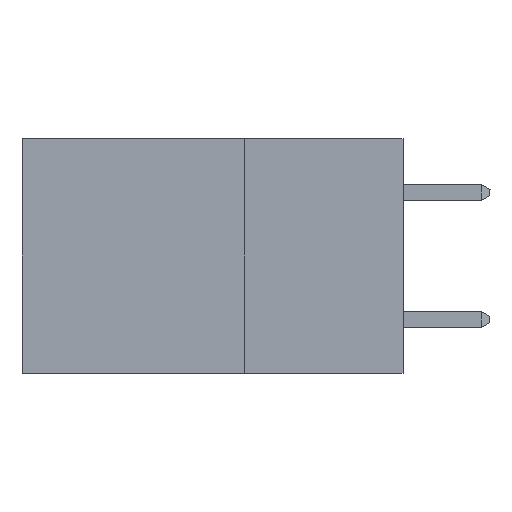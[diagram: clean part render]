
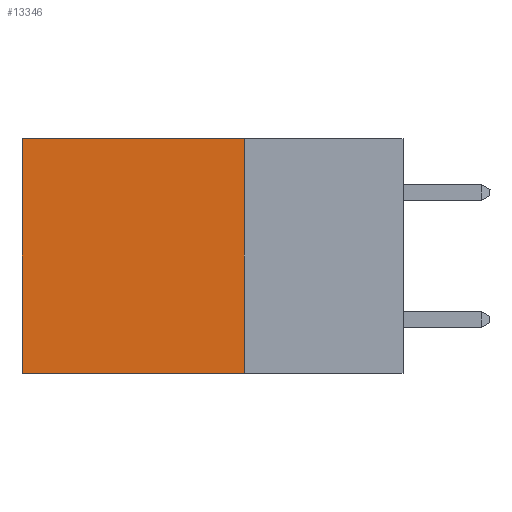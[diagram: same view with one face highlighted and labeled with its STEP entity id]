
A CAD part, left-side view. The second image highlights one B-rep face of the part: STEP entity #13346.
In plain terms, the highlighted planar face has unit normal (-1, 0, 0).
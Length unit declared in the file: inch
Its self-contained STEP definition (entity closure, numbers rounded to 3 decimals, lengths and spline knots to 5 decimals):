
#200 = LINE ( 'NONE', #30138, #27126 ) ;
#284 = LINE ( 'NONE', #18912, #17563 ) ;
#1075 = EDGE_CURVE ( 'NONE', #12666, #24099, #200, .T. ) ;
#2391 = CARTESIAN_POINT ( 'NONE',  ( 0.2875, 0.25, 0. ) ) ;
#2443 = CARTESIAN_POINT ( 'NONE',  ( 0.2875, 0.25, 0. ) ) ;
#2708 = CARTESIAN_POINT ( 'NONE',  ( 0.2875, 0.6, 0. ) ) ;
#4007 = FACE_OUTER_BOUND ( 'NONE', #5356, .T. ) ;
#4535 = VERTEX_POINT ( 'NONE', #2391 ) ;
#5356 = EDGE_LOOP ( 'NONE', ( #16468, #25986, #12578, #10674 ) ) ;
#5748 = VECTOR ( 'NONE', #8883, 39.37008 ) ;
#6306 = PLANE ( 'NONE',  #24813 ) ;
#8027 = CARTESIAN_POINT ( 'NONE',  ( 0.2875, 0.6, -0.37 ) ) ;
#8883 = DIRECTION ( 'NONE',  ( 0., 1., 0. ) ) ;
#10674 = ORIENTED_EDGE ( 'NONE', *, *, #24663, .T. ) ;
#11685 = DIRECTION ( 'NONE',  ( 0., 0., -1. ) ) ;
#12578 = ORIENTED_EDGE ( 'NONE', *, *, #29408, .F. ) ;
#12666 = VERTEX_POINT ( 'NONE', #25464 ) ;
#13307 = DIRECTION ( 'NONE',  ( 1., 0., 0. ) ) ;
#13346 = ADVANCED_FACE ( 'NONE', ( #4007 ), #6306, .F. ) ;
#15611 = CARTESIAN_POINT ( 'NONE',  ( 0.2875, 0.25, 0. ) ) ;
#16468 = ORIENTED_EDGE ( 'NONE', *, *, #23882, .T. ) ;
#17563 = VECTOR ( 'NONE', #19221, 39.37008 ) ;
#18476 = LINE ( 'NONE', #2443, #5748 ) ;
#18912 = CARTESIAN_POINT ( 'NONE',  ( 0.2875, 0.25, 0. ) ) ;
#18998 = CARTESIAN_POINT ( 'NONE',  ( 0.2875, 0.6, 0. ) ) ;
#19221 = DIRECTION ( 'NONE',  ( 0., 0., -1. ) ) ;
#22615 = DIRECTION ( 'NONE',  ( 0., 0., -1. ) ) ;
#23394 = VERTEX_POINT ( 'NONE', #2708 ) ;
#23552 = DIRECTION ( 'NONE',  ( 0., 1., 0. ) ) ;
#23882 = EDGE_CURVE ( 'NONE', #23394, #24099, #25420, .T. ) ;
#24099 = VERTEX_POINT ( 'NONE', #8027 ) ;
#24663 = EDGE_CURVE ( 'NONE', #4535, #23394, #18476, .T. ) ;
#24719 = VECTOR ( 'NONE', #11685, 39.37008 ) ;
#24813 = AXIS2_PLACEMENT_3D ( 'NONE', #15611, #13307, #22615 ) ;
#25420 = LINE ( 'NONE', #18998, #24719 ) ;
#25464 = CARTESIAN_POINT ( 'NONE',  ( 0.2875, 0.25, -0.37 ) ) ;
#25986 = ORIENTED_EDGE ( 'NONE', *, *, #1075, .F. ) ;
#27126 = VECTOR ( 'NONE', #23552, 39.37008 ) ;
#29408 = EDGE_CURVE ( 'NONE', #4535, #12666, #284, .T. ) ;
#30138 = CARTESIAN_POINT ( 'NONE',  ( 0.2875, 0.25, -0.37 ) ) ;
